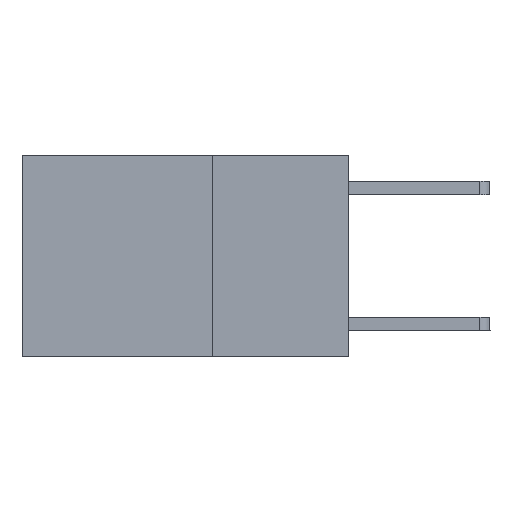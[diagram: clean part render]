
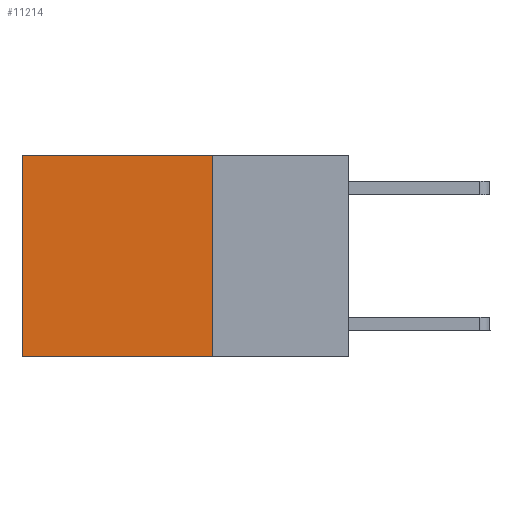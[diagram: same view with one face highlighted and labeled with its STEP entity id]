
A CAD part, left-side view. The second image highlights one B-rep face of the part: STEP entity #11214.
In plain terms, the highlighted planar face has unit normal (-1, 0, 0).
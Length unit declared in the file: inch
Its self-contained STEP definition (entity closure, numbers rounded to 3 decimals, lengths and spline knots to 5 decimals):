
#564 = CARTESIAN_POINT ( 'NONE',  ( 0.2625, 0.25, 0. ) ) ;
#1108 = FACE_OUTER_BOUND ( 'NONE', #10141, .T. ) ;
#1129 = LINE ( 'NONE', #7225, #3611 ) ;
#1553 = CARTESIAN_POINT ( 'NONE',  ( 0.2625, 0.25, -0.37 ) ) ;
#1643 = LINE ( 'NONE', #8061, #3828 ) ;
#1676 = DIRECTION ( 'NONE',  ( 0., 1., 0. ) ) ;
#2097 = VERTEX_POINT ( 'NONE', #3977 ) ;
#2419 = ORIENTED_EDGE ( 'NONE', *, *, #4700, .T. ) ;
#2471 = ORIENTED_EDGE ( 'NONE', *, *, #5228, .F. ) ;
#2500 = ORIENTED_EDGE ( 'NONE', *, *, #6316, .F. ) ;
#2550 = ORIENTED_EDGE ( 'NONE', *, *, #3695, .T. ) ;
#3611 = VECTOR ( 'NONE', #1676, 39.37008 ) ;
#3695 = EDGE_CURVE ( 'NONE', #4526, #3998, #1129, .T. ) ;
#3828 = VECTOR ( 'NONE', #10728, 39.37008 ) ;
#3977 = CARTESIAN_POINT ( 'NONE',  ( 0.2625, 0.6, -0.37 ) ) ;
#3998 = VERTEX_POINT ( 'NONE', #6785 ) ;
#4526 = VERTEX_POINT ( 'NONE', #11011 ) ;
#4700 = EDGE_CURVE ( 'NONE', #3998, #2097, #7050, .T. ) ;
#5228 = EDGE_CURVE ( 'NONE', #10134, #2097, #6452, .T. ) ;
#5254 = DIRECTION ( 'NONE',  ( 0., 0., -1. ) ) ;
#6316 = EDGE_CURVE ( 'NONE', #4526, #10134, #1643, .T. ) ;
#6442 = CARTESIAN_POINT ( 'NONE',  ( 0.2625, 0.25, -0.37 ) ) ;
#6452 = LINE ( 'NONE', #6442, #8597 ) ;
#6541 = DIRECTION ( 'NONE',  ( 0., 0., -1. ) ) ;
#6785 = CARTESIAN_POINT ( 'NONE',  ( 0.2625, 0.6, 0. ) ) ;
#7050 = LINE ( 'NONE', #10994, #9141 ) ;
#7225 = CARTESIAN_POINT ( 'NONE',  ( 0.2625, 0.25, 0. ) ) ;
#7953 = PLANE ( 'NONE',  #10052 ) ;
#8061 = CARTESIAN_POINT ( 'NONE',  ( 0.2625, 0.25, 0. ) ) ;
#8597 = VECTOR ( 'NONE', #11697, 39.37008 ) ;
#9141 = VECTOR ( 'NONE', #6541, 39.37008 ) ;
#10052 = AXIS2_PLACEMENT_3D ( 'NONE', #564, #10660, #5254 ) ;
#10134 = VERTEX_POINT ( 'NONE', #1553 ) ;
#10141 = EDGE_LOOP ( 'NONE', ( #2419, #2471, #2500, #2550 ) ) ;
#10660 = DIRECTION ( 'NONE',  ( 1., 0., 0. ) ) ;
#10728 = DIRECTION ( 'NONE',  ( 0., 0., -1. ) ) ;
#10994 = CARTESIAN_POINT ( 'NONE',  ( 0.2625, 0.6, 0. ) ) ;
#11011 = CARTESIAN_POINT ( 'NONE',  ( 0.2625, 0.25, 0. ) ) ;
#11214 = ADVANCED_FACE ( 'NONE', ( #1108 ), #7953, .F. ) ;
#11697 = DIRECTION ( 'NONE',  ( 0., 1., 0. ) ) ;
